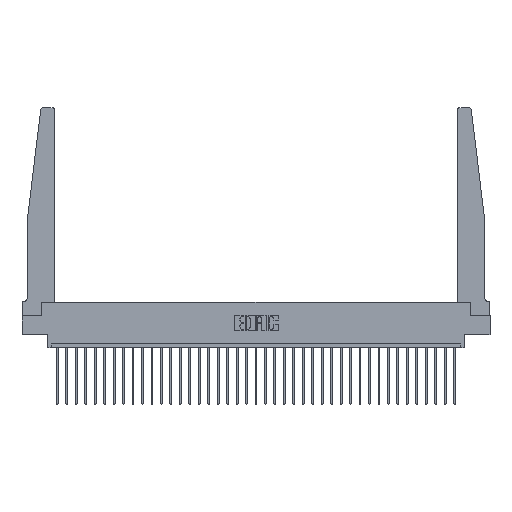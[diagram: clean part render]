
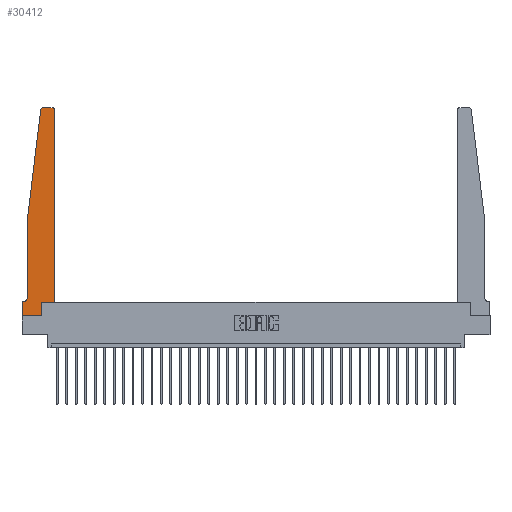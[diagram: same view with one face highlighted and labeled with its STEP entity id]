
A CAD part, top view. The second image highlights one B-rep face of the part: STEP entity #30412.
In plain terms, the highlighted planar face has unit normal (0, 0, 1).
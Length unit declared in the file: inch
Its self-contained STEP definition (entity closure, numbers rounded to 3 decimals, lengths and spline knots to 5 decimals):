
#205 = LINE ( 'NONE', #16613, #24475 ) ;
#796 = ORIENTED_EDGE ( 'NONE', *, *, #31224, .T. ) ;
#1680 = LINE ( 'NONE', #9071, #21071 ) ;
#2451 = LINE ( 'NONE', #18930, #6618 ) ;
#3453 = CARTESIAN_POINT ( 'NONE',  ( 0.065, 1.25, 0.37 ) ) ;
#3732 = CARTESIAN_POINT ( 'NONE',  ( 0.015, 0.1875, 0.37 ) ) ;
#3734 = DIRECTION ( 'NONE',  ( 0., 0., 1. ) ) ;
#4082 = ORIENTED_EDGE ( 'NONE', *, *, #6520, .T. ) ;
#4795 = AXIS2_PLACEMENT_3D ( 'NONE', #6984, #24368, #29074 ) ;
#5082 = CIRCLE ( 'NONE', #10973, 0.03 ) ;
#5097 = EDGE_LOOP ( 'NONE', ( #796, #21284, #26066, #23464, #18826, #12663, #16763, #13323, #21543, #28669, #4082, #24532 ) ) ;
#5199 = EDGE_CURVE ( 'NONE', #13629, #24262, #24707, .T. ) ;
#5894 = DIRECTION ( 'NONE',  ( -0.122, -0.992, 0. ) ) ;
#6175 = DIRECTION ( 'NONE',  ( 1., 0., 0. ) ) ;
#6520 = EDGE_CURVE ( 'NONE', #17384, #23277, #28447, .T. ) ;
#6591 = EDGE_CURVE ( 'NONE', #14884, #16550, #19683, .T. ) ;
#6618 = VECTOR ( 'NONE', #7190, 39.37008 ) ;
#6984 = CARTESIAN_POINT ( 'NONE',  ( 0., 0.1875, 0.37 ) ) ;
#7190 = DIRECTION ( 'NONE',  ( 0., 1., 0. ) ) ;
#7669 = CARTESIAN_POINT ( 'NONE',  ( 0.425, 0.18, 0.37 ) ) ;
#7859 = EDGE_CURVE ( 'NONE', #10560, #17384, #15787, .T. ) ;
#8554 = DIRECTION ( 'NONE',  ( 0., 0., -1. ) ) ;
#8594 = VECTOR ( 'NONE', #12703, 39.37008 ) ;
#9071 = CARTESIAN_POINT ( 'NONE',  ( 0.065, 0.1875, 0.37 ) ) ;
#9073 = EDGE_CURVE ( 'NONE', #26459, #13606, #20253, .T. ) ;
#9084 = EDGE_CURVE ( 'NONE', #23277, #25973, #5082, .T. ) ;
#10206 = DIRECTION ( 'NONE',  ( 1., 0., 0. ) ) ;
#10304 = CARTESIAN_POINT ( 'NONE',  ( 0., 0., 0.37 ) ) ;
#10496 = DIRECTION ( 'NONE',  ( 1., 0., 0. ) ) ;
#10560 = VERTEX_POINT ( 'NONE', #14297 ) ;
#10764 = LINE ( 'NONE', #17435, #14498 ) ;
#10973 = AXIS2_PLACEMENT_3D ( 'NONE', #25584, #3734, #6175 ) ;
#12510 = VECTOR ( 'NONE', #25234, 39.37008 ) ;
#12663 = ORIENTED_EDGE ( 'NONE', *, *, #19240, .T. ) ;
#12703 = DIRECTION ( 'NONE',  ( 1., 0., 0. ) ) ;
#13192 = AXIS2_PLACEMENT_3D ( 'NONE', #30317, #8554, #18467 ) ;
#13323 = ORIENTED_EDGE ( 'NONE', *, *, #20049, .T. ) ;
#13606 = VERTEX_POINT ( 'NONE', #3732 ) ;
#13629 = VERTEX_POINT ( 'NONE', #23353 ) ;
#13804 = LINE ( 'NONE', #10304, #16491 ) ;
#14297 = CARTESIAN_POINT ( 'NONE',  ( 0.2605, 0.18, 0.37 ) ) ;
#14498 = VECTOR ( 'NONE', #27096, 39.37008 ) ;
#14633 = CARTESIAN_POINT ( 'NONE',  ( 0.395, 2.75, 0.37 ) ) ;
#14884 = VERTEX_POINT ( 'NONE', #16090 ) ;
#15037 = CARTESIAN_POINT ( 'NONE',  ( 0.2605, 0., 0.37 ) ) ;
#15634 = DIRECTION ( 'NONE',  ( 0., 1., 0. ) ) ;
#15657 = CARTESIAN_POINT ( 'NONE',  ( 0.27653, 2.72, 0.37 ) ) ;
#15787 = LINE ( 'NONE', #27436, #8594 ) ;
#16072 = AXIS2_PLACEMENT_3D ( 'NONE', #15657, #20201, #10496 ) ;
#16090 = CARTESIAN_POINT ( 'NONE',  ( 0., 0.1875, 0.37 ) ) ;
#16491 = VECTOR ( 'NONE', #10206, 39.37008 ) ;
#16550 = VERTEX_POINT ( 'NONE', #26614 ) ;
#16613 = CARTESIAN_POINT ( 'NONE',  ( 0.065, 1.25, 0.37 ) ) ;
#16763 = ORIENTED_EDGE ( 'NONE', *, *, #6591, .T. ) ;
#16929 = DIRECTION ( 'NONE',  ( 0., -1., 0. ) ) ;
#17384 = VERTEX_POINT ( 'NONE', #7669 ) ;
#17435 = CARTESIAN_POINT ( 'NONE',  ( 0.25, 2.75, 0.37 ) ) ;
#18467 = DIRECTION ( 'NONE',  ( -1., 0., 0. ) ) ;
#18826 = ORIENTED_EDGE ( 'NONE', *, *, #9073, .T. ) ;
#18930 = CARTESIAN_POINT ( 'NONE',  ( 0.2605, 0.18, 0.37 ) ) ;
#19065 = FACE_OUTER_BOUND ( 'NONE', #5097, .T. ) ;
#19240 = EDGE_CURVE ( 'NONE', #13606, #14884, #1680, .T. ) ;
#19582 = EDGE_CURVE ( 'NONE', #30497, #10560, #2451, .T. ) ;
#19620 = EDGE_CURVE ( 'NONE', #20320, #26459, #205, .T. ) ;
#19683 = LINE ( 'NONE', #20364, #12510 ) ;
#20049 = EDGE_CURVE ( 'NONE', #16550, #30497, #13804, .T. ) ;
#20201 = DIRECTION ( 'NONE',  ( 0., 0., 1. ) ) ;
#20253 = CIRCLE ( 'NONE', #13192, 0.05 ) ;
#20320 = VERTEX_POINT ( 'NONE', #26961 ) ;
#20364 = CARTESIAN_POINT ( 'NONE',  ( 0., 0., 0.37 ) ) ;
#20709 = CARTESIAN_POINT ( 'NONE',  ( 0.24675, 2.72367, 0.37 ) ) ;
#21071 = VECTOR ( 'NONE', #21507, 39.37008 ) ;
#21284 = ORIENTED_EDGE ( 'NONE', *, *, #5199, .T. ) ;
#21507 = DIRECTION ( 'NONE',  ( -1., 0., 0. ) ) ;
#21543 = ORIENTED_EDGE ( 'NONE', *, *, #19582, .T. ) ;
#21550 = VECTOR ( 'NONE', #15634, 39.37008 ) ;
#21598 = LINE ( 'NONE', #3453, #30384 ) ;
#22596 = EDGE_CURVE ( 'NONE', #24262, #20320, #21598, .T. ) ;
#23277 = VERTEX_POINT ( 'NONE', #23553 ) ;
#23353 = CARTESIAN_POINT ( 'NONE',  ( 0.27653, 2.75, 0.37 ) ) ;
#23464 = ORIENTED_EDGE ( 'NONE', *, *, #19620, .T. ) ;
#23553 = CARTESIAN_POINT ( 'NONE',  ( 0.425, 2.72, 0.37 ) ) ;
#24262 = VERTEX_POINT ( 'NONE', #20709 ) ;
#24368 = DIRECTION ( 'NONE',  ( 0., 0., 1. ) ) ;
#24475 = VECTOR ( 'NONE', #16929, 39.37008 ) ;
#24532 = ORIENTED_EDGE ( 'NONE', *, *, #9084, .T. ) ;
#24590 = CARTESIAN_POINT ( 'NONE',  ( 0.065, 0.2375, 0.37 ) ) ;
#24707 = CIRCLE ( 'NONE', #16072, 0.03 ) ;
#25234 = DIRECTION ( 'NONE',  ( 0., -1., 0. ) ) ;
#25272 = CARTESIAN_POINT ( 'NONE',  ( 0.425, 0.18, 0.37 ) ) ;
#25584 = CARTESIAN_POINT ( 'NONE',  ( 0.395, 2.72, 0.37 ) ) ;
#25973 = VERTEX_POINT ( 'NONE', #14633 ) ;
#26066 = ORIENTED_EDGE ( 'NONE', *, *, #22596, .T. ) ;
#26459 = VERTEX_POINT ( 'NONE', #24590 ) ;
#26612 = PLANE ( 'NONE',  #4795 ) ;
#26614 = CARTESIAN_POINT ( 'NONE',  ( 0., 0., 0.37 ) ) ;
#26961 = CARTESIAN_POINT ( 'NONE',  ( 0.065, 1.25, 0.37 ) ) ;
#27096 = DIRECTION ( 'NONE',  ( -1., 0., 0. ) ) ;
#27436 = CARTESIAN_POINT ( 'NONE',  ( 0.425, 0.18, 0.37 ) ) ;
#28447 = LINE ( 'NONE', #25272, #21550 ) ;
#28669 = ORIENTED_EDGE ( 'NONE', *, *, #7859, .T. ) ;
#29074 = DIRECTION ( 'NONE',  ( 1., 0., 0. ) ) ;
#30317 = CARTESIAN_POINT ( 'NONE',  ( 0.015, 0.2375, 0.37 ) ) ;
#30384 = VECTOR ( 'NONE', #5894, 39.37008 ) ;
#30412 = ADVANCED_FACE ( 'NONE', ( #19065 ), #26612, .T. ) ;
#30497 = VERTEX_POINT ( 'NONE', #15037 ) ;
#31224 = EDGE_CURVE ( 'NONE', #25973, #13629, #10764, .T. ) ;
